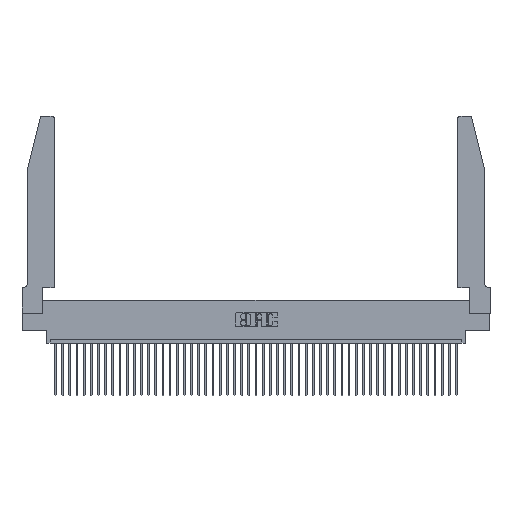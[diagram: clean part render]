
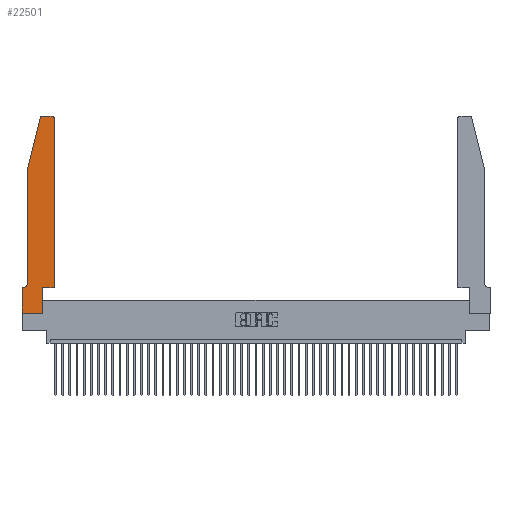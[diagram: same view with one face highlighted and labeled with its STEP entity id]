
A CAD part, top view. The second image highlights one B-rep face of the part: STEP entity #22501.
In plain terms, the highlighted planar face has unit normal (0, 0, 1).
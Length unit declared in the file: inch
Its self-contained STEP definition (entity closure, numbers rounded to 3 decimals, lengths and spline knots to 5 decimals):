
#321 = VECTOR ( 'NONE', #31279, 39.37008 ) ;
#731 = LINE ( 'NONE', #8754, #15723 ) ;
#818 = LINE ( 'NONE', #39587, #9183 ) ;
#1157 = CIRCLE ( 'NONE', #37234, 0.07 ) ;
#1297 = CARTESIAN_POINT ( 'NONE',  ( 0.25487, 2.72718, 0.37 ) ) ;
#1767 = CIRCLE ( 'NONE', #29729, 0.03 ) ;
#2514 = CARTESIAN_POINT ( 'NONE',  ( 0., 0., 0.37 ) ) ;
#3410 = VERTEX_POINT ( 'NONE', #17783 ) ;
#3630 = EDGE_CURVE ( 'NONE', #8547, #37751, #19266, .T. ) ;
#3793 = CARTESIAN_POINT ( 'NONE',  ( 0.4205, 2.72, 0.37 ) ) ;
#4149 = AXIS2_PLACEMENT_3D ( 'NONE', #36134, #9271, #30624 ) ;
#4496 = VERTEX_POINT ( 'NONE', #19472 ) ;
#4868 = CARTESIAN_POINT ( 'NONE',  ( 0.284, 2.72, 0.37 ) ) ;
#6085 = VERTEX_POINT ( 'NONE', #41393 ) ;
#6424 = EDGE_CURVE ( 'NONE', #3410, #8547, #1767, .T. ) ;
#6543 = CARTESIAN_POINT ( 'NONE',  ( 0.0055, 0.35, 0.37 ) ) ;
#6928 = DIRECTION ( 'NONE',  ( 0., 0., 1. ) ) ;
#7033 = LINE ( 'NONE', #8980, #21407 ) ;
#7228 = DIRECTION ( 'NONE',  ( 0., 0., 1. ) ) ;
#7490 = ORIENTED_EDGE ( 'NONE', *, *, #35169, .T. ) ;
#7504 = VECTOR ( 'NONE', #23458, 39.37008 ) ;
#7739 = LINE ( 'NONE', #43170, #26066 ) ;
#8323 = ORIENTED_EDGE ( 'NONE', *, *, #3630, .T. ) ;
#8509 = CARTESIAN_POINT ( 'NONE',  ( 0.2605, 2.75, 0.37 ) ) ;
#8547 = VERTEX_POINT ( 'NONE', #30547 ) ;
#8754 = CARTESIAN_POINT ( 'NONE',  ( 0.0755, 2., 0.37 ) ) ;
#8980 = CARTESIAN_POINT ( 'NONE',  ( 0.4505, 0.35, 0.37 ) ) ;
#9183 = VECTOR ( 'NONE', #18470, 39.37008 ) ;
#9271 = DIRECTION ( 'NONE',  ( 0., 0., 1. ) ) ;
#9371 = VERTEX_POINT ( 'NONE', #6543 ) ;
#10671 = DIRECTION ( 'NONE',  ( 1., 0., 0. ) ) ;
#10981 = VERTEX_POINT ( 'NONE', #12275 ) ;
#11250 = FACE_OUTER_BOUND ( 'NONE', #36335, .T. ) ;
#12275 = CARTESIAN_POINT ( 'NONE',  ( 0.4505, 0.35, 0.37 ) ) ;
#12661 = VERTEX_POINT ( 'NONE', #17278 ) ;
#12668 = ORIENTED_EDGE ( 'NONE', *, *, #36685, .T. ) ;
#14229 = CARTESIAN_POINT ( 'NONE',  ( 0.0755, 0.35, 0.37 ) ) ;
#14683 = EDGE_CURVE ( 'NONE', #23435, #17852, #7739, .T. ) ;
#15219 = DIRECTION ( 'NONE',  ( 0., 1., 0. ) ) ;
#15436 = CARTESIAN_POINT ( 'NONE',  ( 0.4505, 0.35, 0.37 ) ) ;
#15571 = AXIS2_PLACEMENT_3D ( 'NONE', #4868, #7228, #10671 ) ;
#15723 = VECTOR ( 'NONE', #33511, 39.37008 ) ;
#15801 = VERTEX_POINT ( 'NONE', #1297 ) ;
#16413 = LINE ( 'NONE', #14229, #321 ) ;
#17158 = CARTESIAN_POINT ( 'NONE',  ( 0.2865, 0., 0.37 ) ) ;
#17278 = CARTESIAN_POINT ( 'NONE',  ( 0.0755, 0.42, 0.37 ) ) ;
#17766 = CARTESIAN_POINT ( 'NONE',  ( 0.0055, 0.42, 0.37 ) ) ;
#17783 = CARTESIAN_POINT ( 'NONE',  ( 0.4505, 2.72, 0.37 ) ) ;
#17852 = VERTEX_POINT ( 'NONE', #19494 ) ;
#18470 = DIRECTION ( 'NONE',  ( 0., -1., 0. ) ) ;
#18966 = EDGE_CURVE ( 'NONE', #6085, #23435, #41951, .T. ) ;
#19266 = LINE ( 'NONE', #8509, #41397 ) ;
#19472 = CARTESIAN_POINT ( 'NONE',  ( 0.0755, 2., 0.37 ) ) ;
#19494 = CARTESIAN_POINT ( 'NONE',  ( 0.2865, 0.35, 0.37 ) ) ;
#20190 = ORIENTED_EDGE ( 'NONE', *, *, #28085, .T. ) ;
#20771 = EDGE_CURVE ( 'NONE', #4496, #12661, #818, .T. ) ;
#20884 = VERTEX_POINT ( 'NONE', #37408 ) ;
#21407 = VECTOR ( 'NONE', #41138, 39.37008 ) ;
#21593 = DIRECTION ( 'NONE',  ( -1., 0., 0. ) ) ;
#22501 = ADVANCED_FACE ( 'NONE', ( #11250 ), #35827, .T. ) ;
#23435 = VERTEX_POINT ( 'NONE', #17158 ) ;
#23458 = DIRECTION ( 'NONE',  ( 0., -1., 0. ) ) ;
#23504 = EDGE_CURVE ( 'NONE', #12661, #9371, #1157, .T. ) ;
#25254 = LINE ( 'NONE', #2514, #7504 ) ;
#25289 = ORIENTED_EDGE ( 'NONE', *, *, #6424, .T. ) ;
#26066 = VECTOR ( 'NONE', #15219, 39.37008 ) ;
#27819 = CIRCLE ( 'NONE', #15571, 0.03 ) ;
#28085 = EDGE_CURVE ( 'NONE', #15801, #4496, #731, .T. ) ;
#28445 = CARTESIAN_POINT ( 'NONE',  ( 0., 0., 0.37 ) ) ;
#29729 = AXIS2_PLACEMENT_3D ( 'NONE', #3793, #6928, #38440 ) ;
#30190 = DIRECTION ( 'NONE',  ( 1., 0., 0. ) ) ;
#30547 = CARTESIAN_POINT ( 'NONE',  ( 0.4205, 2.75, 0.37 ) ) ;
#30624 = DIRECTION ( 'NONE',  ( 1., 0., 0. ) ) ;
#31279 = DIRECTION ( 'NONE',  ( -1., 0., 0. ) ) ;
#31827 = LINE ( 'NONE', #15436, #37273 ) ;
#32599 = ORIENTED_EDGE ( 'NONE', *, *, #23504, .T. ) ;
#33511 = DIRECTION ( 'NONE',  ( -0.239, -0.971, 0. ) ) ;
#33568 = ORIENTED_EDGE ( 'NONE', *, *, #20771, .T. ) ;
#35169 = EDGE_CURVE ( 'NONE', #10981, #3410, #7033, .T. ) ;
#35270 = ORIENTED_EDGE ( 'NONE', *, *, #35589, .T. ) ;
#35356 = ORIENTED_EDGE ( 'NONE', *, *, #18966, .T. ) ;
#35589 = EDGE_CURVE ( 'NONE', #20884, #6085, #25254, .T. ) ;
#35827 = PLANE ( 'NONE',  #4149 ) ;
#36134 = CARTESIAN_POINT ( 'NONE',  ( 0., 0.35, 0.37 ) ) ;
#36335 = EDGE_LOOP ( 'NONE', ( #8323, #44111, #20190, #33568, #32599, #39659, #35270, #35356, #44558, #12668, #7490, #25289 ) ) ;
#36685 = EDGE_CURVE ( 'NONE', #17852, #10981, #31827, .T. ) ;
#37234 = AXIS2_PLACEMENT_3D ( 'NONE', #17766, #42291, #21593 ) ;
#37273 = VECTOR ( 'NONE', #43726, 39.37008 ) ;
#37408 = CARTESIAN_POINT ( 'NONE',  ( 0., 0.35, 0.37 ) ) ;
#37751 = VERTEX_POINT ( 'NONE', #40543 ) ;
#38440 = DIRECTION ( 'NONE',  ( 1., 0., 0. ) ) ;
#39587 = CARTESIAN_POINT ( 'NONE',  ( 0.0755, 2., 0.37 ) ) ;
#39659 = ORIENTED_EDGE ( 'NONE', *, *, #39951, .T. ) ;
#39951 = EDGE_CURVE ( 'NONE', #9371, #20884, #16413, .T. ) ;
#40543 = CARTESIAN_POINT ( 'NONE',  ( 0.284, 2.75, 0.37 ) ) ;
#41138 = DIRECTION ( 'NONE',  ( 0., 1., 0. ) ) ;
#41393 = CARTESIAN_POINT ( 'NONE',  ( 0., 0., 0.37 ) ) ;
#41397 = VECTOR ( 'NONE', #44585, 39.37008 ) ;
#41951 = LINE ( 'NONE', #28445, #44731 ) ;
#42291 = DIRECTION ( 'NONE',  ( 0., 0., -1. ) ) ;
#43170 = CARTESIAN_POINT ( 'NONE',  ( 0.2865, 0.35, 0.37 ) ) ;
#43726 = DIRECTION ( 'NONE',  ( 1., 0., 0. ) ) ;
#44111 = ORIENTED_EDGE ( 'NONE', *, *, #45811, .T. ) ;
#44558 = ORIENTED_EDGE ( 'NONE', *, *, #14683, .T. ) ;
#44585 = DIRECTION ( 'NONE',  ( -1., 0., 0. ) ) ;
#44731 = VECTOR ( 'NONE', #30190, 39.37008 ) ;
#45811 = EDGE_CURVE ( 'NONE', #37751, #15801, #27819, .T. ) ;
